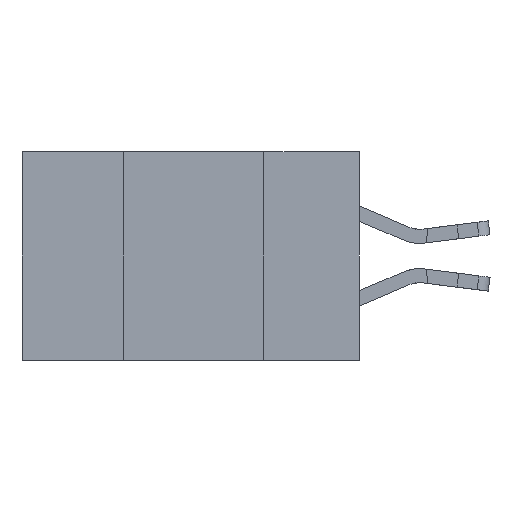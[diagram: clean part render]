
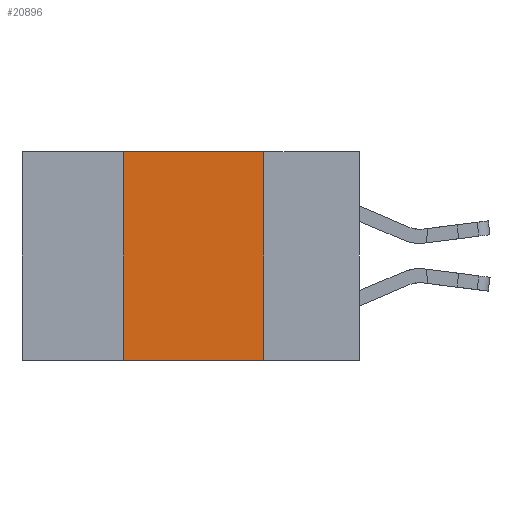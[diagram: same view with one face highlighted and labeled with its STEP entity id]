
A CAD part, left-side view. The second image highlights one B-rep face of the part: STEP entity #20896.
In plain terms, the highlighted planar face has unit normal (-1, 0, 0).
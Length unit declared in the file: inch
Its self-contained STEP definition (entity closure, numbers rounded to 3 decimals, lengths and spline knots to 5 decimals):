
#791 = LINE ( 'NONE', #12943, #4894 ) ;
#914 = CARTESIAN_POINT ( 'NONE',  ( 0., 0.17, -0.37 ) ) ;
#934 = CARTESIAN_POINT ( 'NONE',  ( 0., 0.42, -0.37 ) ) ;
#1191 = CARTESIAN_POINT ( 'NONE',  ( 0., 0.17, 0. ) ) ;
#2298 = CARTESIAN_POINT ( 'NONE',  ( 0., 0.42, 0. ) ) ;
#3465 = ORIENTED_EDGE ( 'NONE', *, *, #8383, .T. ) ;
#4894 = VECTOR ( 'NONE', #16433, 39.37008 ) ;
#5362 = FACE_OUTER_BOUND ( 'NONE', #21948, .T. ) ;
#6516 = ORIENTED_EDGE ( 'NONE', *, *, #11437, .F. ) ;
#6943 = VECTOR ( 'NONE', #13765, 39.37008 ) ;
#7283 = ORIENTED_EDGE ( 'NONE', *, *, #15314, .F. ) ;
#8011 = DIRECTION ( 'NONE',  ( 0., 0., 1. ) ) ;
#8383 = EDGE_CURVE ( 'NONE', #17900, #9708, #791, .T. ) ;
#8923 = VECTOR ( 'NONE', #8011, 39.37008 ) ;
#9708 = VERTEX_POINT ( 'NONE', #914 ) ;
#9946 = DIRECTION ( 'NONE',  ( 1., 0., 0. ) ) ;
#9984 = CARTESIAN_POINT ( 'NONE',  ( 0., 0.6, 0. ) ) ;
#10328 = CARTESIAN_POINT ( 'NONE',  ( 0., 0.17, 0. ) ) ;
#10969 = LINE ( 'NONE', #10328, #6943 ) ;
#11437 = EDGE_CURVE ( 'NONE', #20334, #9708, #10969, .T. ) ;
#11715 = DIRECTION ( 'NONE',  ( 0., -1., 0. ) ) ;
#12943 = CARTESIAN_POINT ( 'NONE',  ( 0., 0.6, -0.37 ) ) ;
#13502 = EDGE_CURVE ( 'NONE', #16583, #20334, #15444, .T. ) ;
#13712 = ORIENTED_EDGE ( 'NONE', *, *, #13502, .F. ) ;
#13765 = DIRECTION ( 'NONE',  ( 0., 0., -1. ) ) ;
#15314 = EDGE_CURVE ( 'NONE', #17900, #16583, #22022, .T. ) ;
#15444 = LINE ( 'NONE', #9984, #19951 ) ;
#15495 = AXIS2_PLACEMENT_3D ( 'NONE', #16780, #9946, #21893 ) ;
#16433 = DIRECTION ( 'NONE',  ( 0., -1., 0. ) ) ;
#16583 = VERTEX_POINT ( 'NONE', #2298 ) ;
#16780 = CARTESIAN_POINT ( 'NONE',  ( 0., 0.6, 0. ) ) ;
#17900 = VERTEX_POINT ( 'NONE', #934 ) ;
#18293 = CARTESIAN_POINT ( 'NONE',  ( 0., 0.42, 0. ) ) ;
#18476 = PLANE ( 'NONE',  #15495 ) ;
#19951 = VECTOR ( 'NONE', #11715, 39.37008 ) ;
#20334 = VERTEX_POINT ( 'NONE', #1191 ) ;
#20896 = ADVANCED_FACE ( 'NONE', ( #5362 ), #18476, .F. ) ;
#21893 = DIRECTION ( 'NONE',  ( 0., 0., -1. ) ) ;
#21948 = EDGE_LOOP ( 'NONE', ( #6516, #13712, #7283, #3465 ) ) ;
#22022 = LINE ( 'NONE', #18293, #8923 ) ;
